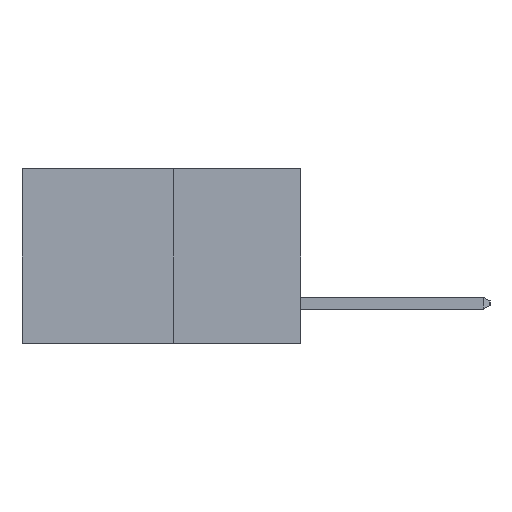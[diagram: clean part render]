
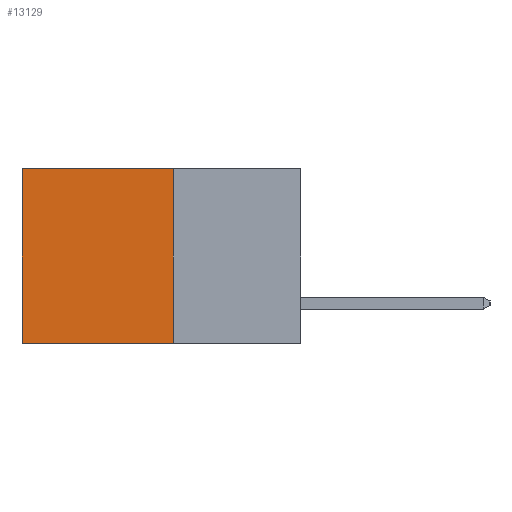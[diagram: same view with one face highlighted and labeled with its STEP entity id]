
A CAD part, left-side view. The second image highlights one B-rep face of the part: STEP entity #13129.
In plain terms, the highlighted planar face has unit normal (-1, 0, 0).
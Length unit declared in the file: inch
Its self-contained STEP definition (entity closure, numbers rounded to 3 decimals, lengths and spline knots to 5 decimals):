
#618 = VERTEX_POINT ( 'NONE', #21787 ) ;
#1321 = PLANE ( 'NONE',  #17098 ) ;
#2555 = LINE ( 'NONE', #16974, #17487 ) ;
#2653 = VERTEX_POINT ( 'NONE', #18300 ) ;
#2676 = VERTEX_POINT ( 'NONE', #7487 ) ;
#3226 = EDGE_CURVE ( 'NONE', #2676, #2653, #20515, .T. ) ;
#3353 = DIRECTION ( 'NONE',  ( 1., 0., 0. ) ) ;
#3667 = CARTESIAN_POINT ( 'NONE',  ( 0.277, 0.27, -0.37 ) ) ;
#4241 = EDGE_CURVE ( 'NONE', #618, #2676, #2555, .T. ) ;
#5049 = DIRECTION ( 'NONE',  ( 0., 0., -1. ) ) ;
#7487 = CARTESIAN_POINT ( 'NONE',  ( 0.277, 0.59, 0. ) ) ;
#7918 = CARTESIAN_POINT ( 'NONE',  ( 0.277, 0.59, -0.37 ) ) ;
#8421 = VECTOR ( 'NONE', #17309, 39.37008 ) ;
#9196 = CARTESIAN_POINT ( 'NONE',  ( 0.277, 0.27, -0.37 ) ) ;
#9357 = VERTEX_POINT ( 'NONE', #21806 ) ;
#9450 = CARTESIAN_POINT ( 'NONE',  ( 0.277, 0.27, -0.37 ) ) ;
#9624 = ORIENTED_EDGE ( 'NONE', *, *, #24112, .F. ) ;
#10405 = EDGE_CURVE ( 'NONE', #9357, #2653, #12986, .T. ) ;
#11453 = DIRECTION ( 'NONE',  ( 0., 0., -1. ) ) ;
#12963 = ORIENTED_EDGE ( 'NONE', *, *, #10405, .F. ) ;
#12986 = LINE ( 'NONE', #3667, #8421 ) ;
#13129 = ADVANCED_FACE ( 'NONE', ( #22452 ), #1321, .F. ) ;
#16765 = EDGE_LOOP ( 'NONE', ( #24627, #12963, #9624, #17811 ) ) ;
#16974 = CARTESIAN_POINT ( 'NONE',  ( 0.277, 0.27, 0. ) ) ;
#16993 = DIRECTION ( 'NONE',  ( 0., 0., -1. ) ) ;
#17027 = DIRECTION ( 'NONE',  ( 0., 1., 0. ) ) ;
#17098 = AXIS2_PLACEMENT_3D ( 'NONE', #9196, #3353, #16993 ) ;
#17309 = DIRECTION ( 'NONE',  ( 0., 1., 0. ) ) ;
#17487 = VECTOR ( 'NONE', #17027, 39.37008 ) ;
#17811 = ORIENTED_EDGE ( 'NONE', *, *, #4241, .T. ) ;
#17949 = VECTOR ( 'NONE', #11453, 39.37008 ) ;
#18300 = CARTESIAN_POINT ( 'NONE',  ( 0.277, 0.59, -0.37 ) ) ;
#18535 = LINE ( 'NONE', #9450, #17949 ) ;
#20515 = LINE ( 'NONE', #7918, #24984 ) ;
#21787 = CARTESIAN_POINT ( 'NONE',  ( 0.277, 0.27, 0. ) ) ;
#21806 = CARTESIAN_POINT ( 'NONE',  ( 0.277, 0.27, -0.37 ) ) ;
#22452 = FACE_OUTER_BOUND ( 'NONE', #16765, .T. ) ;
#24112 = EDGE_CURVE ( 'NONE', #618, #9357, #18535, .T. ) ;
#24627 = ORIENTED_EDGE ( 'NONE', *, *, #3226, .T. ) ;
#24984 = VECTOR ( 'NONE', #5049, 39.37008 ) ;
